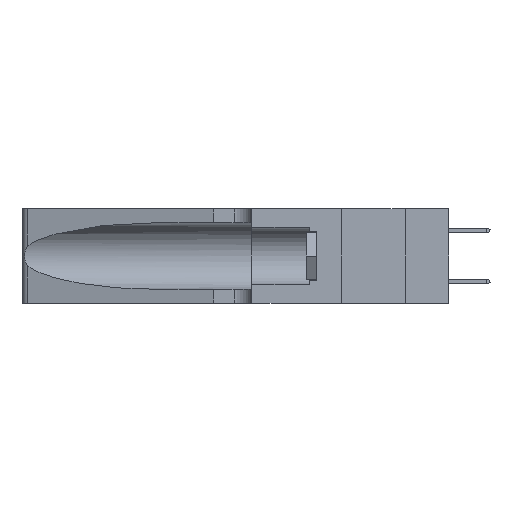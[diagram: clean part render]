
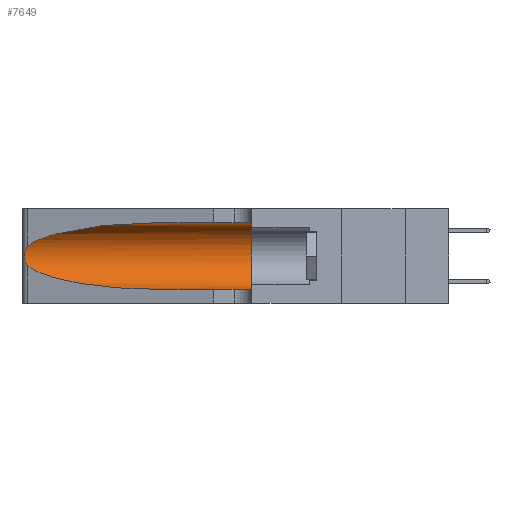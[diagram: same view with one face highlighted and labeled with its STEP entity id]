
A CAD part, left-side view. The second image highlights one B-rep face of the part: STEP entity #7649.
In plain terms, the highlighted cylindrical face has radius 3.308 mm (diameter 6.617 mm), a partial arc.
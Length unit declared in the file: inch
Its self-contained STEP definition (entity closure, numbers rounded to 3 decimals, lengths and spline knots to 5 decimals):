
#379 = CARTESIAN_POINT ( 'NONE',  ( 0.25789, 1.23486, 0.15765 ) ) ;
#862 = CYLINDRICAL_SURFACE ( 'NONE', #13703, 0.13025 ) ;
#899 = CARTESIAN_POINT ( 'NONE',  ( 0.18966, 0.96281, 0.31525 ) ) ;
#1844 = CARTESIAN_POINT ( 'NONE',  ( 0.25487, 1.22718, 0.22369 ) ) ;
#2904 = CARTESIAN_POINT ( 'NONE',  ( 0.25639, 1.23184, 0.21858 ) ) ;
#3398 = CARTESIAN_POINT ( 'NONE',  ( 0.1305, 0.72297, 0.31525 ) ) ;
#3820 = ORIENTED_EDGE ( 'NONE', *, *, #19103, .T. ) ;
#4494 = CARTESIAN_POINT ( 'NONE',  ( 0.18966, 0.96281, 0.05475 ) ) ;
#5009 = CARTESIAN_POINT ( 'NONE',  ( 0.1305, 0.72297, 0.05475 ) ) ;
#5670 = CARTESIAN_POINT ( 'NONE',  ( 0.2373, 1.15595, 0.28018 ) ) ;
#5942 = CARTESIAN_POINT ( 'NONE',  ( 0.1305, 1.61858, 0.05475 ) ) ;
#6846 = EDGE_CURVE ( 'NONE', #29315, #29027, #25816, .T. ) ;
#6993 = EDGE_CURVE ( 'NONE', #29315, #13381, #18419, .T. ) ;
#7057 = CARTESIAN_POINT ( 'NONE',  ( 0.25487, 1.22718, 0.14631 ) ) ;
#7343 = CARTESIAN_POINT ( 'NONE',  ( 0.25854, 1.2359, 0.20912 ) ) ;
#7391 = AXIS2_PLACEMENT_3D ( 'NONE', #18877, #26204, #14389 ) ;
#7536 = CARTESIAN_POINT ( 'NONE',  ( 0.26075, 1.23896, 0.19203 ) ) ;
#7649 = ADVANCED_FACE ( 'NONE', ( #27987 ), #862, .F. ) ;
#7711 = CARTESIAN_POINT ( 'NONE',  ( 0.1305, 1.61858, 0.185 ) ) ;
#7915 = DIRECTION ( 'NONE',  ( 0., 0., -1. ) ) ;
#9203 = CARTESIAN_POINT ( 'NONE',  ( 0.1305, 0.35, 0.31525 ) ) ;
#9841 = VERTEX_POINT ( 'NONE', #5009 ) ;
#9900 = CARTESIAN_POINT ( 'NONE',  ( 0.26018, 1.23835, 0.19895 ) ) ;
#10191 = B_SPLINE_CURVE_WITH_KNOTS ( 'NONE', 3,
 ( #12402, #26711, #2904, #28973, #7343, #9900, #7536, #28873, #29629, #26493, #379, #17728, #19503, #14478 ),
 .UNSPECIFIED., .F., .F.,
 ( 4, 2, 2, 2, 2, 2, 4 ),
 ( 0., 0.00027, 0.00053, 0.00107, 0.0016, 0.00187, 0.00214 ),
 .UNSPECIFIED. ) ;
#10369 = CARTESIAN_POINT ( 'NONE',  ( 0.25487, 1.22718, 0.14631 ) ) ;
#11505 = EDGE_CURVE ( 'NONE', #29027, #30553, #15821, .T. ) ;
#11598 = EDGE_CURVE ( 'NONE', #13381, #28623, #10191, .T. ) ;
#12402 = CARTESIAN_POINT ( 'NONE',  ( 0.25487, 1.22718, 0.22369 ) ) ;
#13279 = EDGE_LOOP ( 'NONE', ( #15538, #19589, #29700, #3820, #16744, #18667 ) ) ;
#13381 = VERTEX_POINT ( 'NONE', #1844 ) ;
#13703 = AXIS2_PLACEMENT_3D ( 'NONE', #7711, #14861, #7915 ) ;
#14389 = DIRECTION ( 'NONE',  ( 0., 0., 1. ) ) ;
#14478 = CARTESIAN_POINT ( 'NONE',  ( 0.25487, 1.22718, 0.14631 ) ) ;
#14861 = DIRECTION ( 'NONE',  ( 0., -1., 0. ) ) ;
#15231 = CARTESIAN_POINT ( 'NONE',  ( 0.1305, 1.61858, 0.31525 ) ) ;
#15538 = ORIENTED_EDGE ( 'NONE', *, *, #6993, .T. ) ;
#15582 = DIRECTION ( 'NONE',  ( 0., -1., 0. ) ) ;
#15734 = LINE ( 'NONE', #5942, #20233 ) ;
#15821 = CIRCLE ( 'NONE', #7391, 0.13025 ) ;
#16041 = VECTOR ( 'NONE', #20152, 39.37008 ) ;
#16076 = CARTESIAN_POINT ( 'NONE',  ( 0.2373, 1.15595, 0.08982 ) ) ;
#16744 = ORIENTED_EDGE ( 'NONE', *, *, #11505, .F. ) ;
#17728 = CARTESIAN_POINT ( 'NONE',  ( 0.25639, 1.23186, 0.15144 ) ) ;
#18419 =( BOUNDED_CURVE ( )  B_SPLINE_CURVE ( 3, ( #3398, #899, #5670, #29598 ),
 .UNSPECIFIED., .F., .F. ) 
 B_SPLINE_CURVE_WITH_KNOTS ( ( 4, 4 ),
 ( 1.5708, 2.84003 ),
 .UNSPECIFIED. ) 
 CURVE ( )  GEOMETRIC_REPRESENTATION_ITEM ( )  RATIONAL_B_SPLINE_CURVE ( ( 1., 0.87, 0.87, 1. ) ) 
 REPRESENTATION_ITEM ( '' )  );
#18667 = ORIENTED_EDGE ( 'NONE', *, *, #6846, .F. ) ;
#18677 = CARTESIAN_POINT ( 'NONE',  ( 0.1305, 0.35, 0.05475 ) ) ;
#18877 = CARTESIAN_POINT ( 'NONE',  ( 0.1305, 0.35, 0.185 ) ) ;
#19103 = EDGE_CURVE ( 'NONE', #9841, #30553, #15734, .T. ) ;
#19503 = CARTESIAN_POINT ( 'NONE',  ( 0.25555, 1.22993, 0.14849 ) ) ;
#19589 = ORIENTED_EDGE ( 'NONE', *, *, #11598, .T. ) ;
#20152 = DIRECTION ( 'NONE',  ( 0., -1., 0. ) ) ;
#20233 = VECTOR ( 'NONE', #15582, 39.37008 ) ;
#23416 = CARTESIAN_POINT ( 'NONE',  ( 0.1305, 0.72297, 0.05475 ) ) ;
#24625 = CARTESIAN_POINT ( 'NONE',  ( 0.1305, 0.72297, 0.31525 ) ) ;
#24687 = EDGE_CURVE ( 'NONE', #28623, #9841, #24947, .T. ) ;
#24947 =( BOUNDED_CURVE ( )  B_SPLINE_CURVE ( 3, ( #7057, #16076, #4494, #23416 ),
 .UNSPECIFIED., .F., .F. ) 
 B_SPLINE_CURVE_WITH_KNOTS ( ( 4, 4 ),
 ( 3.44316, 4.71239 ),
 .UNSPECIFIED. ) 
 CURVE ( )  GEOMETRIC_REPRESENTATION_ITEM ( )  RATIONAL_B_SPLINE_CURVE ( ( 1., 0.87, 0.87, 1. ) ) 
 REPRESENTATION_ITEM ( '' )  );
#25816 = LINE ( 'NONE', #15231, #16041 ) ;
#26204 = DIRECTION ( 'NONE',  ( 0., 1., 0. ) ) ;
#26493 = CARTESIAN_POINT ( 'NONE',  ( 0.25856, 1.23593, 0.16098 ) ) ;
#26711 = CARTESIAN_POINT ( 'NONE',  ( 0.25555, 1.22994, 0.2215 ) ) ;
#27987 = FACE_OUTER_BOUND ( 'NONE', #13279, .T. ) ;
#28623 = VERTEX_POINT ( 'NONE', #10369 ) ;
#28873 = CARTESIAN_POINT ( 'NONE',  ( 0.26075, 1.23896, 0.178 ) ) ;
#28973 = CARTESIAN_POINT ( 'NONE',  ( 0.25787, 1.23484, 0.2124 ) ) ;
#29027 = VERTEX_POINT ( 'NONE', #9203 ) ;
#29315 = VERTEX_POINT ( 'NONE', #24625 ) ;
#29598 = CARTESIAN_POINT ( 'NONE',  ( 0.25487, 1.22718, 0.22369 ) ) ;
#29629 = CARTESIAN_POINT ( 'NONE',  ( 0.26017, 1.23833, 0.17102 ) ) ;
#29700 = ORIENTED_EDGE ( 'NONE', *, *, #24687, .T. ) ;
#30553 = VERTEX_POINT ( 'NONE', #18677 ) ;
